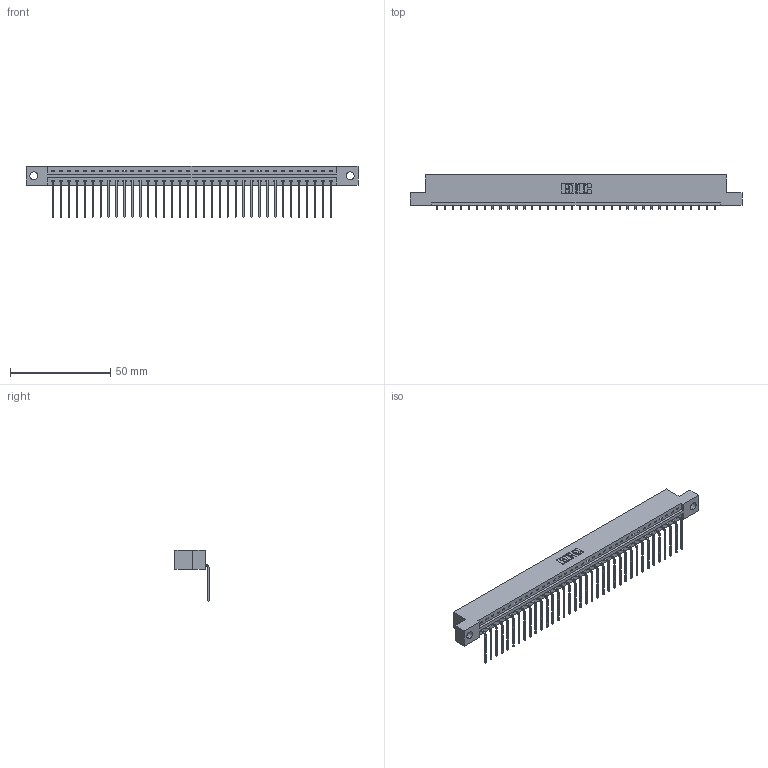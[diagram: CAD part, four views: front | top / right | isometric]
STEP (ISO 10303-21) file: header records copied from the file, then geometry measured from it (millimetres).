
FILE_DESCRIPTION (( 'STEP AP203' ), '1' );
FILE_NAME ('387-036-559-104.STEP', '2018-09-19T01:40:31', ( '' ), ( '' ), 'SwSTEP 2.0', 'SolidWorks 2016', '' );
FILE_SCHEMA (( 'CONFIG_CONTROL_DESIGN' ));
Length unit declared in the file: inch
Products named in the file (3): 337 Part_Flush Mounting Lugs - 0.156 Dia-TH; 345-292-001_558 559 Tail - 1; 387-036-559-104
Assembly tree (37 placements, depth 2):
  387-036-559-104
    337 Part_Flush Mounting Lugs - 0.156 Dia-TH
    345-292-001_558 559 Tail - 1  x36
Bounding box: 165.66 x 17.09 x 25.53 mm (x, y, z)
Volume: 17174.5 mm3; surface area: 18246.1 mm2
Topology: 37 solids, 37 shells, 2418 faces, 7295 edges, 4814 vertices
Faces by surface type: plane 1798, cylinder 620
Entity records: 27623 total; most frequent: CARTESIAN_POINT 4818, ORIENTED_EDGE 4790, DIRECTION 4067, EDGE_CURVE 2395, LINE 2267, VECTOR 2267, VERTEX_POINT 1594, AXIS2_PLACEMENT_3D 900
